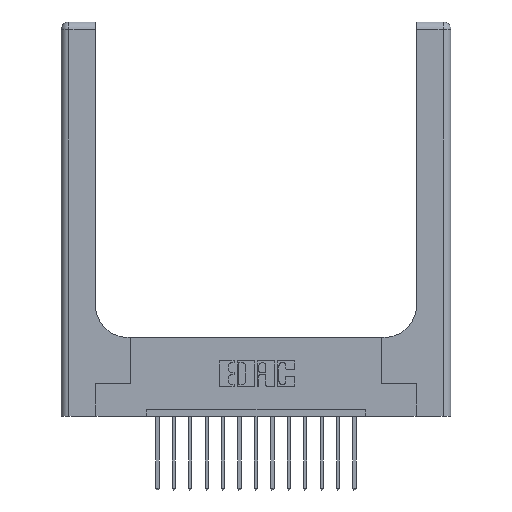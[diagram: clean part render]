
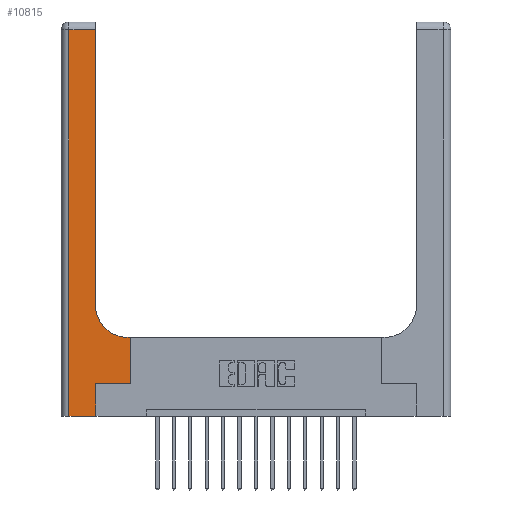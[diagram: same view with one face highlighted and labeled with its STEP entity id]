
A CAD part, top view. The second image highlights one B-rep face of the part: STEP entity #10815.
In plain terms, the highlighted planar face has unit normal (0, 0, 1).
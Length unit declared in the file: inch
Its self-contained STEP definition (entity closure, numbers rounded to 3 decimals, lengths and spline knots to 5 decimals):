
#88 = DIRECTION ( 'NONE',  ( 1., 0., 0. ) ) ;
#468 = EDGE_CURVE ( 'NONE', #13494, #5876, #15285, .T. ) ;
#601 = ORIENTED_EDGE ( 'NONE', *, *, #12985, .T. ) ;
#794 = ORIENTED_EDGE ( 'NONE', *, *, #13986, .T. ) ;
#945 = VECTOR ( 'NONE', #17258, 39.37008 ) ;
#1060 = CARTESIAN_POINT ( 'NONE',  ( 0.06, 3., 0.37 ) ) ;
#1486 = AXIS2_PLACEMENT_3D ( 'NONE', #2384, #16116, #3915 ) ;
#1553 = CARTESIAN_POINT ( 'NONE',  ( 0.528, 0.25, 0.37 ) ) ;
#1634 = LINE ( 'NONE', #1553, #4877 ) ;
#2384 = CARTESIAN_POINT ( 'NONE',  ( 0.51, 0.85, 0.37 ) ) ;
#2385 = VECTOR ( 'NONE', #88, 39.37008 ) ;
#2444 = LINE ( 'NONE', #9398, #4784 ) ;
#2467 = VECTOR ( 'NONE', #3532, 39.37008 ) ;
#2635 = VERTEX_POINT ( 'NONE', #9861 ) ;
#2801 = VECTOR ( 'NONE', #14982, 39.37008 ) ;
#2852 = VERTEX_POINT ( 'NONE', #9485 ) ;
#2981 = EDGE_CURVE ( 'NONE', #3178, #2852, #10088, .T. ) ;
#3178 = VERTEX_POINT ( 'NONE', #15978 ) ;
#3532 = DIRECTION ( 'NONE',  ( 0., 1., 0. ) ) ;
#3915 = DIRECTION ( 'NONE',  ( 1., 0., 0. ) ) ;
#3917 = LINE ( 'NONE', #1060, #945 ) ;
#4102 = CARTESIAN_POINT ( 'NONE',  ( 0., 0., 0.37 ) ) ;
#4298 = CARTESIAN_POINT ( 'NONE',  ( 0.06, 2.94, 0.37 ) ) ;
#4355 = ORIENTED_EDGE ( 'NONE', *, *, #7410, .T. ) ;
#4442 = ORIENTED_EDGE ( 'NONE', *, *, #16884, .T. ) ;
#4580 = VERTEX_POINT ( 'NONE', #4298 ) ;
#4784 = VECTOR ( 'NONE', #7883, 39.37008 ) ;
#4865 = LINE ( 'NONE', #15737, #2467 ) ;
#4877 = VECTOR ( 'NONE', #6896, 39.37008 ) ;
#5035 = CARTESIAN_POINT ( 'NONE',  ( 0.51, 0.6, 0.37 ) ) ;
#5247 = LINE ( 'NONE', #4102, #2385 ) ;
#5876 = VERTEX_POINT ( 'NONE', #5035 ) ;
#6896 = DIRECTION ( 'NONE',  ( 0., 1., 0. ) ) ;
#6955 = LINE ( 'NONE', #16674, #2801 ) ;
#7041 = EDGE_CURVE ( 'NONE', #2635, #3178, #2444, .T. ) ;
#7123 = CARTESIAN_POINT ( 'NONE',  ( 0.06, 0., 0.37 ) ) ;
#7410 = EDGE_CURVE ( 'NONE', #17577, #4580, #6955, .T. ) ;
#7792 = FACE_OUTER_BOUND ( 'NONE', #12286, .T. ) ;
#7883 = DIRECTION ( 'NONE',  ( 0., 1., 0. ) ) ;
#8031 = ORIENTED_EDGE ( 'NONE', *, *, #7041, .T. ) ;
#9308 = CARTESIAN_POINT ( 'NONE',  ( 0., 3., 0.37 ) ) ;
#9398 = CARTESIAN_POINT ( 'NONE',  ( 0.265, 0., 0.37 ) ) ;
#9485 = CARTESIAN_POINT ( 'NONE',  ( 0.528, 0.25, 0.37 ) ) ;
#9861 = CARTESIAN_POINT ( 'NONE',  ( 0.265, 0., 0.37 ) ) ;
#10088 = LINE ( 'NONE', #11441, #12876 ) ;
#10561 = PLANE ( 'NONE',  #14273 ) ;
#10815 = ADVANCED_FACE ( 'NONE', ( #7792 ), #10561, .F. ) ;
#10837 = EDGE_CURVE ( 'NONE', #2852, #13494, #1634, .T. ) ;
#11276 = ORIENTED_EDGE ( 'NONE', *, *, #468, .T. ) ;
#11400 = VECTOR ( 'NONE', #14306, 39.37008 ) ;
#11441 = CARTESIAN_POINT ( 'NONE',  ( 0.265, 0.25, 0.37 ) ) ;
#12286 = EDGE_LOOP ( 'NONE', ( #4442, #4355, #794, #15607, #8031, #12947, #13782, #11276, #601 ) ) ;
#12346 = VERTEX_POINT ( 'NONE', #7123 ) ;
#12632 = CARTESIAN_POINT ( 'NONE',  ( 0.26, 0.85, 0.37 ) ) ;
#12787 = CARTESIAN_POINT ( 'NONE',  ( 0.26, 0.6, 0.37 ) ) ;
#12876 = VECTOR ( 'NONE', #15521, 39.37008 ) ;
#12947 = ORIENTED_EDGE ( 'NONE', *, *, #2981, .T. ) ;
#12985 = EDGE_CURVE ( 'NONE', #5876, #14394, #13713, .T. ) ;
#13244 = DIRECTION ( 'NONE',  ( 0., 0., -1. ) ) ;
#13494 = VERTEX_POINT ( 'NONE', #14365 ) ;
#13713 = CIRCLE ( 'NONE', #1486, 0.25 ) ;
#13751 = CARTESIAN_POINT ( 'NONE',  ( 0.26, 2.94, 0.37 ) ) ;
#13782 = ORIENTED_EDGE ( 'NONE', *, *, #10837, .T. ) ;
#13986 = EDGE_CURVE ( 'NONE', #4580, #12346, #3917, .T. ) ;
#14273 = AXIS2_PLACEMENT_3D ( 'NONE', #9308, #13244, #17317 ) ;
#14306 = DIRECTION ( 'NONE',  ( -1., 0., 0. ) ) ;
#14365 = CARTESIAN_POINT ( 'NONE',  ( 0.528, 0.6, 0.37 ) ) ;
#14394 = VERTEX_POINT ( 'NONE', #12632 ) ;
#14982 = DIRECTION ( 'NONE',  ( -1., 0., 0. ) ) ;
#15043 = EDGE_CURVE ( 'NONE', #12346, #2635, #5247, .T. ) ;
#15285 = LINE ( 'NONE', #12787, #11400 ) ;
#15521 = DIRECTION ( 'NONE',  ( 1., 0., 0. ) ) ;
#15607 = ORIENTED_EDGE ( 'NONE', *, *, #15043, .T. ) ;
#15737 = CARTESIAN_POINT ( 'NONE',  ( 0.26, 3., 0.37 ) ) ;
#15978 = CARTESIAN_POINT ( 'NONE',  ( 0.265, 0.25, 0.37 ) ) ;
#16116 = DIRECTION ( 'NONE',  ( 0., 0., -1. ) ) ;
#16674 = CARTESIAN_POINT ( 'NONE',  ( 0., 2.94, 0.37 ) ) ;
#16884 = EDGE_CURVE ( 'NONE', #14394, #17577, #4865, .T. ) ;
#17258 = DIRECTION ( 'NONE',  ( 0., -1., 0. ) ) ;
#17317 = DIRECTION ( 'NONE',  ( -1., 0., 0. ) ) ;
#17577 = VERTEX_POINT ( 'NONE', #13751 ) ;
